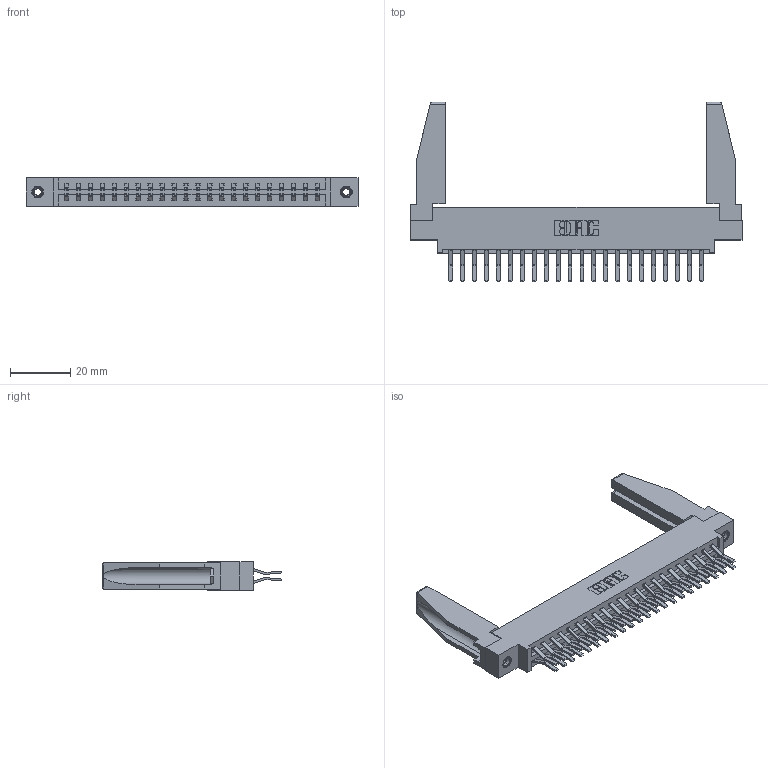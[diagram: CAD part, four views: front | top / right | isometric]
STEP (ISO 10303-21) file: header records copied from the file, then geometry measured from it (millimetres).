
FILE_DESCRIPTION (( 'STEP AP203' ), '1' );
FILE_NAME ('337-044-560-878.STEP', '2019-10-11T14:08:34', ( '' ), ( '' ), 'SwSTEP 2.0', 'SolidWorks 2016', '' );
FILE_SCHEMA (( 'CONFIG_CONTROL_DESIGN' ));
Length unit declared in the file: inch
Products named in the file (5): 345-292-001_560 Tail; 337-044-560-878; 345-250-001_345-250-001-102; 307-220-078; 337 Part_0.170 Offset - 0.156 Dia-TI
Assembly tree (49 placements, depth 2):
  337-044-560-878
    337 Part_0.170 Offset - 0.156 Dia-TI
    345-292-001_560 Tail  x44
    345-250-001_345-250-001-102  x2
    307-220-078  x2
Bounding box: 110.19 x 59.58 x 9.4 mm (x, y, z)
Volume: 15510.2 mm3; surface area: 17598.6 mm2
Topology: 49 solids, 49 shells, 2712 faces, 8001 edges, 5266 vertices
Faces by surface type: plane 1830, cylinder 866, cone 12, torus 4
Entity records: 22304 total; most frequent: CARTESIAN_POINT 3776, ORIENTED_EDGE 3668, DIRECTION 3258, EDGE_CURVE 1834, LINE 1664, VECTOR 1664, VERTEX_POINT 1216, AXIS2_PLACEMENT_3D 797
